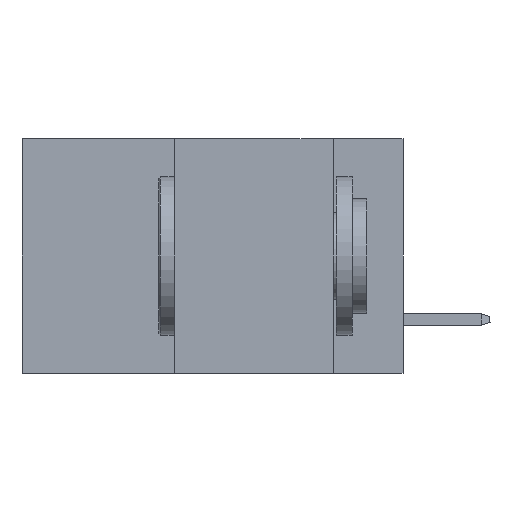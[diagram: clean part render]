
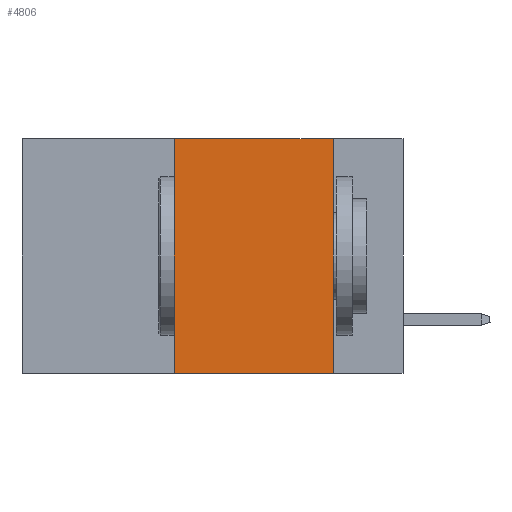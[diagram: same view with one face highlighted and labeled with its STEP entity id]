
A CAD part, left-side view. The second image highlights one B-rep face of the part: STEP entity #4806.
In plain terms, the highlighted planar face has unit normal (-1, 0, 0).
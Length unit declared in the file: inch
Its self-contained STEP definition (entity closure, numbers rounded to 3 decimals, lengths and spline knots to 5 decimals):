
#128 = CARTESIAN_POINT ( 'NONE',  ( 0., 0.6, -0.37 ) ) ;
#1139 = ORIENTED_EDGE ( 'NONE', *, *, #25481, .F. ) ;
#1666 = CARTESIAN_POINT ( 'NONE',  ( 0., 0.11, -0.37 ) ) ;
#1946 = EDGE_LOOP ( 'NONE', ( #4545, #8495, #1139, #32073 ) ) ;
#2796 = CARTESIAN_POINT ( 'NONE',  ( 0., 0.36, -0.37 ) ) ;
#2870 = FACE_OUTER_BOUND ( 'NONE', #1946, .T. ) ;
#3074 = LINE ( 'NONE', #16349, #24481 ) ;
#4545 = ORIENTED_EDGE ( 'NONE', *, *, #33139, .F. ) ;
#4806 = ADVANCED_FACE ( 'NONE', ( #2870 ), #10325, .F. ) ;
#4817 = LINE ( 'NONE', #33126, #32105 ) ;
#5621 = VECTOR ( 'NONE', #22816, 39.37008 ) ;
#5853 = VECTOR ( 'NONE', #8337, 39.37008 ) ;
#5910 = DIRECTION ( 'NONE',  ( 1., 0., 0. ) ) ;
#6122 = CARTESIAN_POINT ( 'NONE',  ( 0., 0.6, 0. ) ) ;
#7306 = CARTESIAN_POINT ( 'NONE',  ( 0., 0.11, 0. ) ) ;
#7618 = VERTEX_POINT ( 'NONE', #7306 ) ;
#8337 = DIRECTION ( 'NONE',  ( 0., -1., 0. ) ) ;
#8495 = ORIENTED_EDGE ( 'NONE', *, *, #18712, .F. ) ;
#10325 = PLANE ( 'NONE',  #18228 ) ;
#13967 = EDGE_CURVE ( 'NONE', #21642, #24227, #26237, .T. ) ;
#16146 = CARTESIAN_POINT ( 'NONE',  ( 0., 0.36, 0. ) ) ;
#16349 = CARTESIAN_POINT ( 'NONE',  ( 0., 0.11, 0. ) ) ;
#18228 = AXIS2_PLACEMENT_3D ( 'NONE', #24015, #5910, #20771 ) ;
#18712 = EDGE_CURVE ( 'NONE', #26545, #7618, #21653, .T. ) ;
#20771 = DIRECTION ( 'NONE',  ( 0., 0., -1. ) ) ;
#21642 = VERTEX_POINT ( 'NONE', #2796 ) ;
#21653 = LINE ( 'NONE', #6122, #5853 ) ;
#22816 = DIRECTION ( 'NONE',  ( 0., -1., 0. ) ) ;
#23086 = DIRECTION ( 'NONE',  ( 0., 0., 1. ) ) ;
#24015 = CARTESIAN_POINT ( 'NONE',  ( 0., 0.6, 0. ) ) ;
#24227 = VERTEX_POINT ( 'NONE', #1666 ) ;
#24481 = VECTOR ( 'NONE', #29190, 39.37008 ) ;
#25481 = EDGE_CURVE ( 'NONE', #21642, #26545, #4817, .T. ) ;
#26237 = LINE ( 'NONE', #128, #5621 ) ;
#26545 = VERTEX_POINT ( 'NONE', #16146 ) ;
#29190 = DIRECTION ( 'NONE',  ( 0., 0., -1. ) ) ;
#32073 = ORIENTED_EDGE ( 'NONE', *, *, #13967, .T. ) ;
#32105 = VECTOR ( 'NONE', #23086, 39.37008 ) ;
#33126 = CARTESIAN_POINT ( 'NONE',  ( 0., 0.36, 0. ) ) ;
#33139 = EDGE_CURVE ( 'NONE', #7618, #24227, #3074, .T. ) ;
